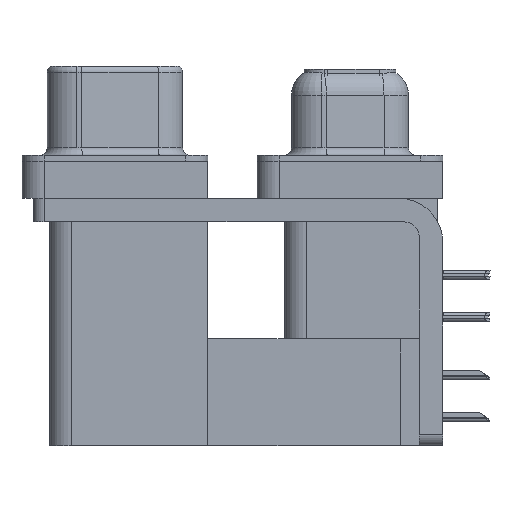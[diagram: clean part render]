
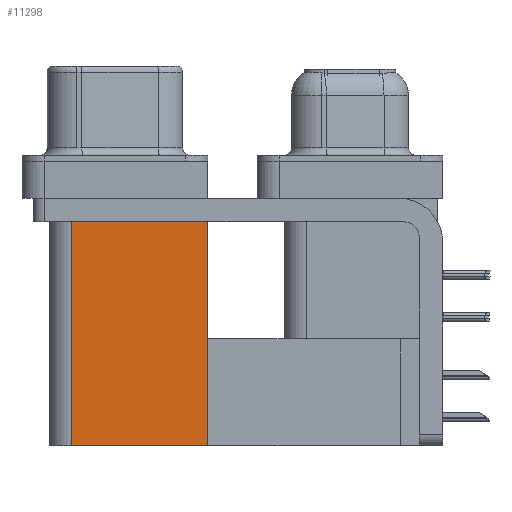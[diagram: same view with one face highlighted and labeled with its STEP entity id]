
A CAD part, left-side view. The second image highlights one B-rep face of the part: STEP entity #11298.
In plain terms, the highlighted planar face has unit normal (-1, 0, 0).
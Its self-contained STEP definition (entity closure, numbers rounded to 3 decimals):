
#1278 = CARTESIAN_POINT ( 'NONE',  ( 3.7, 9.6, -19.2 ) ) ;
#2875 = VERTEX_POINT ( 'NONE', #50584 ) ;
#3530 = EDGE_LOOP ( 'NONE', ( #18210, #16582, #28924, #7919 ) ) ;
#4473 = EDGE_CURVE ( 'NONE', #49769, #2875, #51427, .T. ) ;
#6287 = FACE_OUTER_BOUND ( 'NONE', #3530, .T. ) ;
#7364 = VECTOR ( 'NONE', #35785, 1000. ) ;
#7919 = ORIENTED_EDGE ( 'NONE', *, *, #4473, .T. ) ;
#8323 = DIRECTION ( 'NONE',  ( 0., 0., 1. ) ) ;
#10545 = CARTESIAN_POINT ( 'NONE',  ( 3.7, 18.8, -19.2 ) ) ;
#10844 = CARTESIAN_POINT ( 'NONE',  ( 3.7, 9.6, -19.2 ) ) ;
#11298 = ADVANCED_FACE ( 'NONE', ( #6287 ), #34420, .F. ) ;
#11607 = CARTESIAN_POINT ( 'NONE',  ( 3.7, 9.6, -2.5 ) ) ;
#13801 = VECTOR ( 'NONE', #8323, 1000. ) ;
#16582 = ORIENTED_EDGE ( 'NONE', *, *, #37536, .F. ) ;
#18210 = ORIENTED_EDGE ( 'NONE', *, *, #19681, .T. ) ;
#18257 = VERTEX_POINT ( 'NONE', #10545 ) ;
#18322 = CARTESIAN_POINT ( 'NONE',  ( 3.7, 9.6, -19.2 ) ) ;
#18466 = DIRECTION ( 'NONE',  ( 0., 0., -1. ) ) ;
#19622 = VECTOR ( 'NONE', #27041, 1000. ) ;
#19681 = EDGE_CURVE ( 'NONE', #2875, #45614, #35516, .T. ) ;
#27041 = DIRECTION ( 'NONE',  ( 0., 1., 0. ) ) ;
#28146 = AXIS2_PLACEMENT_3D ( 'NONE', #1278, #41860, #18466 ) ;
#28924 = ORIENTED_EDGE ( 'NONE', *, *, #49226, .F. ) ;
#29330 = LINE ( 'NONE', #32497, #13801 ) ;
#31394 = CARTESIAN_POINT ( 'NONE',  ( 3.7, 18.8, -2.5 ) ) ;
#32497 = CARTESIAN_POINT ( 'NONE',  ( 3.7, 18.8, -19.2 ) ) ;
#33629 = VECTOR ( 'NONE', #34938, 1000. ) ;
#34420 = PLANE ( 'NONE',  #28146 ) ;
#34938 = DIRECTION ( 'NONE',  ( 0., 1., 0. ) ) ;
#35516 = LINE ( 'NONE', #11607, #19622 ) ;
#35785 = DIRECTION ( 'NONE',  ( 0., 0., 1. ) ) ;
#37536 = EDGE_CURVE ( 'NONE', #18257, #45614, #29330, .T. ) ;
#41860 = DIRECTION ( 'NONE',  ( 1., 0., 0. ) ) ;
#42380 = LINE ( 'NONE', #43145, #33629 ) ;
#43145 = CARTESIAN_POINT ( 'NONE',  ( 3.7, 9.6, -19.2 ) ) ;
#45614 = VERTEX_POINT ( 'NONE', #31394 ) ;
#49226 = EDGE_CURVE ( 'NONE', #49769, #18257, #42380, .T. ) ;
#49769 = VERTEX_POINT ( 'NONE', #18322 ) ;
#50584 = CARTESIAN_POINT ( 'NONE',  ( 3.7, 9.6, -2.5 ) ) ;
#51427 = LINE ( 'NONE', #10844, #7364 ) ;
